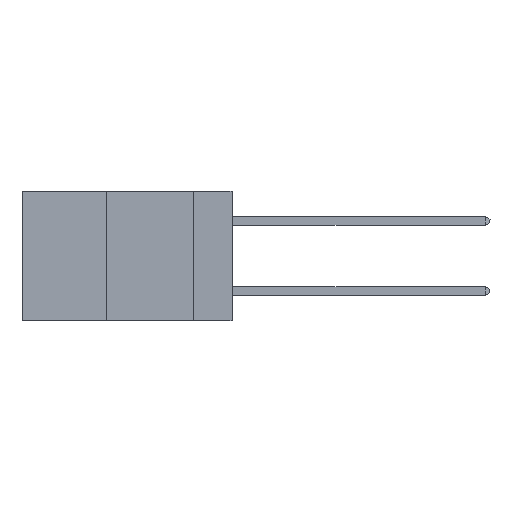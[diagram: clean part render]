
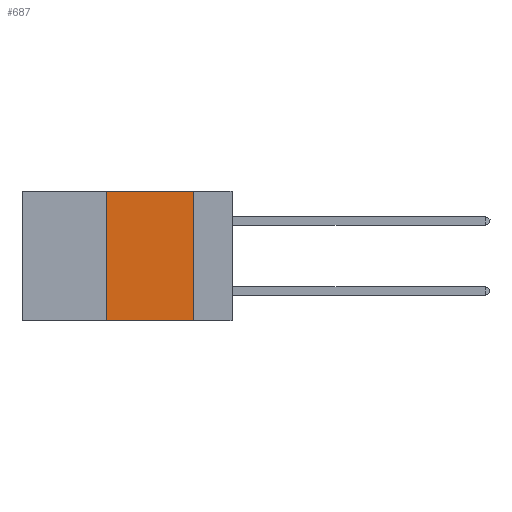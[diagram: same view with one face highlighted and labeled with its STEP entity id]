
A CAD part, left-side view. The second image highlights one B-rep face of the part: STEP entity #687.
In plain terms, the highlighted planar face has unit normal (-1, 0, 0).
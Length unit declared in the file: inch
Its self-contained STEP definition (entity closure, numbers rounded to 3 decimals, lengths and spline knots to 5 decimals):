
#687 = ADVANCED_FACE ( 'NONE', ( #29635 ), #33960, .F. ) ;
#1497 = LINE ( 'NONE', #35234, #26513 ) ;
#3749 = DIRECTION ( 'NONE',  ( 0., 0., 1. ) ) ;
#4841 = VERTEX_POINT ( 'NONE', #40835 ) ;
#7574 = CARTESIAN_POINT ( 'NONE',  ( 0., 0.11, 0. ) ) ;
#8364 = ORIENTED_EDGE ( 'NONE', *, *, #32849, .T. ) ;
#8722 = VERTEX_POINT ( 'NONE', #38343 ) ;
#9940 = CARTESIAN_POINT ( 'NONE',  ( 0., 0.36, 0. ) ) ;
#11054 = ORIENTED_EDGE ( 'NONE', *, *, #18769, .F. ) ;
#14063 = EDGE_CURVE ( 'NONE', #16221, #32368, #1497, .T. ) ;
#14906 = CARTESIAN_POINT ( 'NONE',  ( 0., 0.6, 0. ) ) ;
#15045 = DIRECTION ( 'NONE',  ( 0., 0., -1. ) ) ;
#16221 = VERTEX_POINT ( 'NONE', #7574 ) ;
#16385 = EDGE_LOOP ( 'NONE', ( #34136, #35558, #11054, #8364 ) ) ;
#18769 = EDGE_CURVE ( 'NONE', #8722, #4841, #40355, .T. ) ;
#21873 = DIRECTION ( 'NONE',  ( 0., -1., 0. ) ) ;
#21949 = CARTESIAN_POINT ( 'NONE',  ( 0., 0.6, -0.37 ) ) ;
#24544 = LINE ( 'NONE', #21949, #34025 ) ;
#25014 = DIRECTION ( 'NONE',  ( 0., -1., 0. ) ) ;
#25218 = VECTOR ( 'NONE', #21873, 39.37008 ) ;
#26513 = VECTOR ( 'NONE', #36767, 39.37008 ) ;
#29635 = FACE_OUTER_BOUND ( 'NONE', #16385, .T. ) ;
#30888 = DIRECTION ( 'NONE',  ( 1., 0., 0. ) ) ;
#32368 = VERTEX_POINT ( 'NONE', #35222 ) ;
#32849 = EDGE_CURVE ( 'NONE', #8722, #32368, #24544, .T. ) ;
#33675 = LINE ( 'NONE', #40809, #25218 ) ;
#33960 = PLANE ( 'NONE',  #40153 ) ;
#34025 = VECTOR ( 'NONE', #25014, 39.37008 ) ;
#34136 = ORIENTED_EDGE ( 'NONE', *, *, #14063, .F. ) ;
#35222 = CARTESIAN_POINT ( 'NONE',  ( 0., 0.11, -0.37 ) ) ;
#35234 = CARTESIAN_POINT ( 'NONE',  ( 0., 0.11, 0. ) ) ;
#35558 = ORIENTED_EDGE ( 'NONE', *, *, #38152, .F. ) ;
#36767 = DIRECTION ( 'NONE',  ( 0., 0., -1. ) ) ;
#36889 = VECTOR ( 'NONE', #3749, 39.37008 ) ;
#38152 = EDGE_CURVE ( 'NONE', #4841, #16221, #33675, .T. ) ;
#38343 = CARTESIAN_POINT ( 'NONE',  ( 0., 0.36, -0.37 ) ) ;
#40153 = AXIS2_PLACEMENT_3D ( 'NONE', #14906, #30888, #15045 ) ;
#40355 = LINE ( 'NONE', #9940, #36889 ) ;
#40809 = CARTESIAN_POINT ( 'NONE',  ( 0., 0.6, 0. ) ) ;
#40835 = CARTESIAN_POINT ( 'NONE',  ( 0., 0.36, 0. ) ) ;
